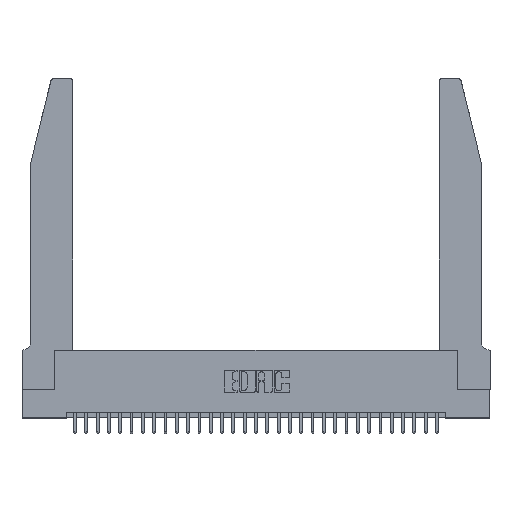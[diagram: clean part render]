
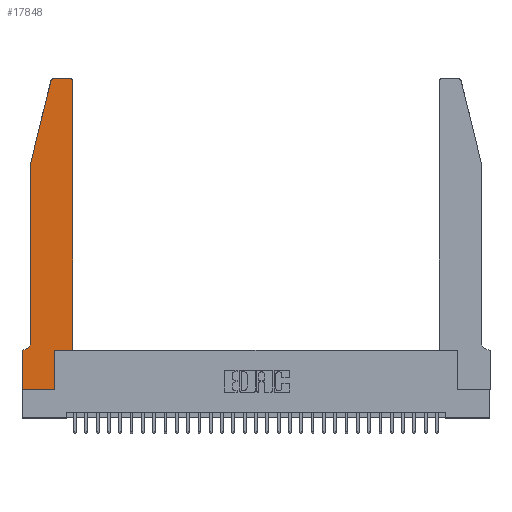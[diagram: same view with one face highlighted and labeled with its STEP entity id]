
A CAD part, top view. The second image highlights one B-rep face of the part: STEP entity #17848.
In plain terms, the highlighted planar face has unit normal (0, 0, 1).
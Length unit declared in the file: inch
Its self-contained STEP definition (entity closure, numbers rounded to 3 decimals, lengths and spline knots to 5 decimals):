
#519 = LINE ( 'NONE', #17232, #26044 ) ;
#589 = LINE ( 'NONE', #17629, #31779 ) ;
#684 = VECTOR ( 'NONE', #11447, 39.37008 ) ;
#761 = CARTESIAN_POINT ( 'NONE',  ( 0.0055, 0.35, 0.37 ) ) ;
#840 = CARTESIAN_POINT ( 'NONE',  ( 0.2865, 0.35, 0.37 ) ) ;
#1128 = DIRECTION ( 'NONE',  ( -1., 0., 0. ) ) ;
#1428 = LINE ( 'NONE', #14164, #20438 ) ;
#1957 = LINE ( 'NONE', #15918, #27428 ) ;
#2369 = EDGE_CURVE ( 'NONE', #18048, #30258, #31352, .T. ) ;
#2435 = DIRECTION ( 'NONE',  ( 0., 0., 1. ) ) ;
#2746 = DIRECTION ( 'NONE',  ( 1., 0., 0. ) ) ;
#2862 = CARTESIAN_POINT ( 'NONE',  ( 0., 0.35, 0.37 ) ) ;
#3320 = ORIENTED_EDGE ( 'NONE', *, *, #27925, .T. ) ;
#4076 = EDGE_CURVE ( 'NONE', #11424, #22513, #1957, .T. ) ;
#4259 = EDGE_CURVE ( 'NONE', #17028, #21524, #10540, .T. ) ;
#4272 = DIRECTION ( 'NONE',  ( -1., 0., 0. ) ) ;
#4699 = EDGE_CURVE ( 'NONE', #22513, #19423, #23570, .T. ) ;
#5285 = EDGE_CURVE ( 'NONE', #12258, #18048, #7354, .T. ) ;
#6160 = CARTESIAN_POINT ( 'NONE',  ( 0.2865, 0., 0.37 ) ) ;
#6198 = DIRECTION ( 'NONE',  ( 0., 0., 1. ) ) ;
#7115 = VERTEX_POINT ( 'NONE', #840 ) ;
#7354 = LINE ( 'NONE', #7866, #684 ) ;
#7537 = CARTESIAN_POINT ( 'NONE',  ( 0.284, 2.75, 0.37 ) ) ;
#7555 = PLANE ( 'NONE',  #23245 ) ;
#7866 = CARTESIAN_POINT ( 'NONE',  ( 0.0755, 2., 0.37 ) ) ;
#8225 = CARTESIAN_POINT ( 'NONE',  ( 0., 0., 0.37 ) ) ;
#8667 = CARTESIAN_POINT ( 'NONE',  ( 0.0755, 0.35, 0.37 ) ) ;
#9112 = CARTESIAN_POINT ( 'NONE',  ( 0.4505, 0.35, 0.37 ) ) ;
#9402 = FACE_OUTER_BOUND ( 'NONE', #21703, .T. ) ;
#9482 = ORIENTED_EDGE ( 'NONE', *, *, #4076, .T. ) ;
#9898 = ORIENTED_EDGE ( 'NONE', *, *, #18442, .T. ) ;
#10054 = DIRECTION ( 'NONE',  ( 0., 0., 1. ) ) ;
#10168 = AXIS2_PLACEMENT_3D ( 'NONE', #17329, #2435, #19795 ) ;
#10540 = LINE ( 'NONE', #9112, #22828 ) ;
#11078 = ORIENTED_EDGE ( 'NONE', *, *, #11207, .T. ) ;
#11207 = EDGE_CURVE ( 'NONE', #21524, #17968, #15435, .T. ) ;
#11236 = CARTESIAN_POINT ( 'NONE',  ( 0.4505, 2.72, 0.37 ) ) ;
#11424 = VERTEX_POINT ( 'NONE', #2862 ) ;
#11447 = DIRECTION ( 'NONE',  ( -0.239, -0.971, 0. ) ) ;
#11556 = ORIENTED_EDGE ( 'NONE', *, *, #20743, .T. ) ;
#12106 = CIRCLE ( 'NONE', #15455, 0.07 ) ;
#12258 = VERTEX_POINT ( 'NONE', #23679 ) ;
#12525 = DIRECTION ( 'NONE',  ( 0., 0., -1. ) ) ;
#12880 = AXIS2_PLACEMENT_3D ( 'NONE', #20962, #6198, #23423 ) ;
#13076 = EDGE_CURVE ( 'NONE', #19423, #7115, #519, .T. ) ;
#13671 = CARTESIAN_POINT ( 'NONE',  ( 0.0755, 2., 0.37 ) ) ;
#14164 = CARTESIAN_POINT ( 'NONE',  ( 0.2605, 2.75, 0.37 ) ) ;
#14755 = DIRECTION ( 'NONE',  ( 0., 1., 0. ) ) ;
#15400 = ORIENTED_EDGE ( 'NONE', *, *, #2369, .T. ) ;
#15435 = CIRCLE ( 'NONE', #10168, 0.03 ) ;
#15455 = AXIS2_PLACEMENT_3D ( 'NONE', #27180, #12525, #29605 ) ;
#15644 = CARTESIAN_POINT ( 'NONE',  ( 0.0755, 2., 0.37 ) ) ;
#15918 = CARTESIAN_POINT ( 'NONE',  ( 0., 0., 0.37 ) ) ;
#16117 = DIRECTION ( 'NONE',  ( 0., -1., 0. ) ) ;
#16251 = EDGE_CURVE ( 'NONE', #18027, #11424, #17861, .T. ) ;
#16553 = DIRECTION ( 'NONE',  ( 0., 1., 0. ) ) ;
#17025 = CARTESIAN_POINT ( 'NONE',  ( 0.0755, 0.42, 0.37 ) ) ;
#17028 = VERTEX_POINT ( 'NONE', #23636 ) ;
#17068 = VECTOR ( 'NONE', #30275, 39.37008 ) ;
#17104 = VECTOR ( 'NONE', #1128, 39.37008 ) ;
#17232 = CARTESIAN_POINT ( 'NONE',  ( 0.2865, 0.35, 0.37 ) ) ;
#17329 = CARTESIAN_POINT ( 'NONE',  ( 0.4205, 2.72, 0.37 ) ) ;
#17510 = ORIENTED_EDGE ( 'NONE', *, *, #16251, .T. ) ;
#17574 = ORIENTED_EDGE ( 'NONE', *, *, #4259, .T. ) ;
#17629 = CARTESIAN_POINT ( 'NONE',  ( 0.4505, 0.35, 0.37 ) ) ;
#17848 = ADVANCED_FACE ( 'NONE', ( #9402 ), #7555, .T. ) ;
#17861 = LINE ( 'NONE', #8667, #17104 ) ;
#17968 = VERTEX_POINT ( 'NONE', #30047 ) ;
#18027 = VERTEX_POINT ( 'NONE', #761 ) ;
#18048 = VERTEX_POINT ( 'NONE', #15644 ) ;
#18442 = EDGE_CURVE ( 'NONE', #30258, #18027, #12106, .T. ) ;
#19274 = ORIENTED_EDGE ( 'NONE', *, *, #5285, .T. ) ;
#19423 = VERTEX_POINT ( 'NONE', #6160 ) ;
#19795 = DIRECTION ( 'NONE',  ( 1., 0., 0. ) ) ;
#20438 = VECTOR ( 'NONE', #4272, 39.37008 ) ;
#20743 = EDGE_CURVE ( 'NONE', #7115, #17028, #589, .T. ) ;
#20962 = CARTESIAN_POINT ( 'NONE',  ( 0.284, 2.72, 0.37 ) ) ;
#21524 = VERTEX_POINT ( 'NONE', #11236 ) ;
#21680 = CIRCLE ( 'NONE', #12880, 0.03 ) ;
#21703 = EDGE_LOOP ( 'NONE', ( #29516, #3320, #19274, #15400, #9898, #17510, #9482, #28249, #26329, #11556, #17574, #11078 ) ) ;
#22513 = VERTEX_POINT ( 'NONE', #29340 ) ;
#22828 = VECTOR ( 'NONE', #16553, 39.37008 ) ;
#23245 = AXIS2_PLACEMENT_3D ( 'NONE', #24783, #10054, #27222 ) ;
#23309 = DIRECTION ( 'NONE',  ( 0., -1., 0. ) ) ;
#23368 = VECTOR ( 'NONE', #16117, 39.37008 ) ;
#23423 = DIRECTION ( 'NONE',  ( 1., 0., 0. ) ) ;
#23570 = LINE ( 'NONE', #8225, #17068 ) ;
#23636 = CARTESIAN_POINT ( 'NONE',  ( 0.4505, 0.35, 0.37 ) ) ;
#23679 = CARTESIAN_POINT ( 'NONE',  ( 0.25487, 2.72718, 0.37 ) ) ;
#24783 = CARTESIAN_POINT ( 'NONE',  ( 0., 0.35, 0.37 ) ) ;
#26044 = VECTOR ( 'NONE', #14755, 39.37008 ) ;
#26329 = ORIENTED_EDGE ( 'NONE', *, *, #13076, .T. ) ;
#27180 = CARTESIAN_POINT ( 'NONE',  ( 0.0055, 0.42, 0.37 ) ) ;
#27222 = DIRECTION ( 'NONE',  ( 1., 0., 0. ) ) ;
#27428 = VECTOR ( 'NONE', #23309, 39.37008 ) ;
#27925 = EDGE_CURVE ( 'NONE', #29707, #12258, #21680, .T. ) ;
#28249 = ORIENTED_EDGE ( 'NONE', *, *, #4699, .T. ) ;
#29340 = CARTESIAN_POINT ( 'NONE',  ( 0., 0., 0.37 ) ) ;
#29503 = EDGE_CURVE ( 'NONE', #17968, #29707, #1428, .T. ) ;
#29516 = ORIENTED_EDGE ( 'NONE', *, *, #29503, .T. ) ;
#29605 = DIRECTION ( 'NONE',  ( -1., 0., 0. ) ) ;
#29707 = VERTEX_POINT ( 'NONE', #7537 ) ;
#30047 = CARTESIAN_POINT ( 'NONE',  ( 0.4205, 2.75, 0.37 ) ) ;
#30258 = VERTEX_POINT ( 'NONE', #17025 ) ;
#30275 = DIRECTION ( 'NONE',  ( 1., 0., 0. ) ) ;
#31352 = LINE ( 'NONE', #13671, #23368 ) ;
#31779 = VECTOR ( 'NONE', #2746, 39.37008 ) ;
